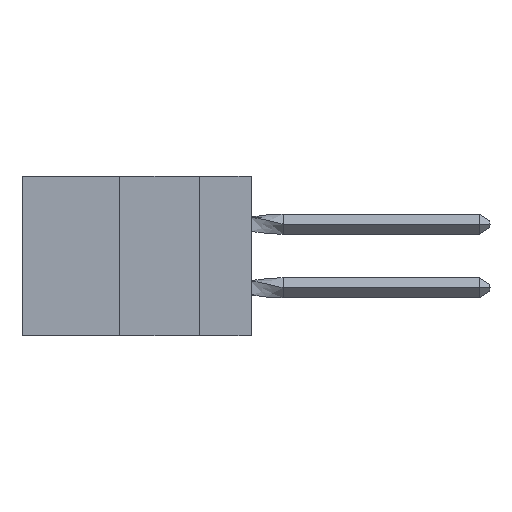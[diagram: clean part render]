
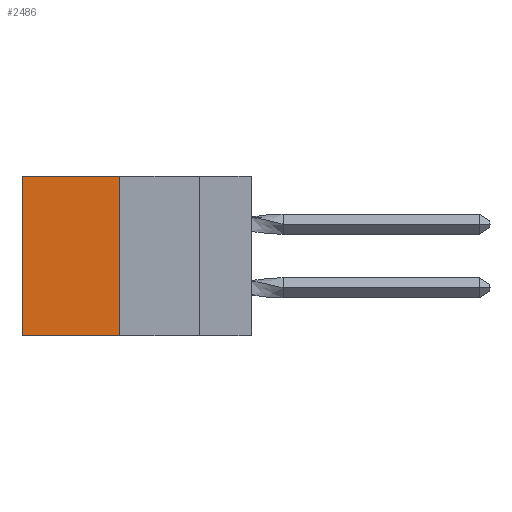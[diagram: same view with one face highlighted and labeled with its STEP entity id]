
A CAD part, left-side view. The second image highlights one B-rep face of the part: STEP entity #2486.
In plain terms, the highlighted planar face has unit normal (-1, 0, 0).
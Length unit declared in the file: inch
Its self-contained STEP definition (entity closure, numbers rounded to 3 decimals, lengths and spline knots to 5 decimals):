
#429 = LINE ( 'NONE', #14163, #9256 ) ;
#598 = DIRECTION ( 'NONE',  ( 0., 0., -1. ) ) ;
#746 = ORIENTED_EDGE ( 'NONE', *, *, #4108, .F. ) ;
#756 = EDGE_CURVE ( 'NONE', #1989, #4097, #17853, .T. ) ;
#1416 = DIRECTION ( 'NONE',  ( 0., 0., -1. ) ) ;
#1487 = PLANE ( 'NONE',  #18151 ) ;
#1989 = VERTEX_POINT ( 'NONE', #10812 ) ;
#2200 = FACE_OUTER_BOUND ( 'NONE', #18125, .T. ) ;
#2486 = ADVANCED_FACE ( 'NONE', ( #2200 ), #1487, .F. ) ;
#3358 = DIRECTION ( 'NONE',  ( 0., 1., 0. ) ) ;
#3598 = CARTESIAN_POINT ( 'NONE',  ( 0.305, 0.72, -0.5 ) ) ;
#3675 = VERTEX_POINT ( 'NONE', #11292 ) ;
#4078 = CARTESIAN_POINT ( 'NONE',  ( 0.305, 0.413, 0. ) ) ;
#4097 = VERTEX_POINT ( 'NONE', #13686 ) ;
#4108 = EDGE_CURVE ( 'NONE', #7511, #4097, #11448, .T. ) ;
#5016 = ORIENTED_EDGE ( 'NONE', *, *, #17165, .F. ) ;
#5124 = DIRECTION ( 'NONE',  ( 0., 0., -1. ) ) ;
#7511 = VERTEX_POINT ( 'NONE', #18015 ) ;
#9074 = DIRECTION ( 'NONE',  ( 1., 0., 0. ) ) ;
#9250 = CARTESIAN_POINT ( 'NONE',  ( 0.305, 0.413, -0.5 ) ) ;
#9256 = VECTOR ( 'NONE', #598, 39.37008 ) ;
#9391 = EDGE_CURVE ( 'NONE', #3675, #1989, #19242, .T. ) ;
#10812 = CARTESIAN_POINT ( 'NONE',  ( 0.305, 0.72, 0. ) ) ;
#10963 = ORIENTED_EDGE ( 'NONE', *, *, #9391, .T. ) ;
#11292 = CARTESIAN_POINT ( 'NONE',  ( 0.305, 0.413, 0. ) ) ;
#11448 = LINE ( 'NONE', #9250, #13536 ) ;
#12019 = CARTESIAN_POINT ( 'NONE',  ( 0.305, 0.413, -0.5 ) ) ;
#13536 = VECTOR ( 'NONE', #3358, 39.37008 ) ;
#13686 = CARTESIAN_POINT ( 'NONE',  ( 0.305, 0.72, -0.5 ) ) ;
#14163 = CARTESIAN_POINT ( 'NONE',  ( 0.305, 0.413, -0.5 ) ) ;
#15536 = ORIENTED_EDGE ( 'NONE', *, *, #756, .T. ) ;
#15823 = DIRECTION ( 'NONE',  ( 0., 1., 0. ) ) ;
#15985 = VECTOR ( 'NONE', #5124, 39.37008 ) ;
#17165 = EDGE_CURVE ( 'NONE', #3675, #7511, #429, .T. ) ;
#17853 = LINE ( 'NONE', #3598, #15985 ) ;
#18015 = CARTESIAN_POINT ( 'NONE',  ( 0.305, 0.413, -0.5 ) ) ;
#18125 = EDGE_LOOP ( 'NONE', ( #15536, #746, #5016, #10963 ) ) ;
#18151 = AXIS2_PLACEMENT_3D ( 'NONE', #12019, #9074, #1416 ) ;
#19005 = VECTOR ( 'NONE', #15823, 39.37008 ) ;
#19242 = LINE ( 'NONE', #4078, #19005 ) ;
